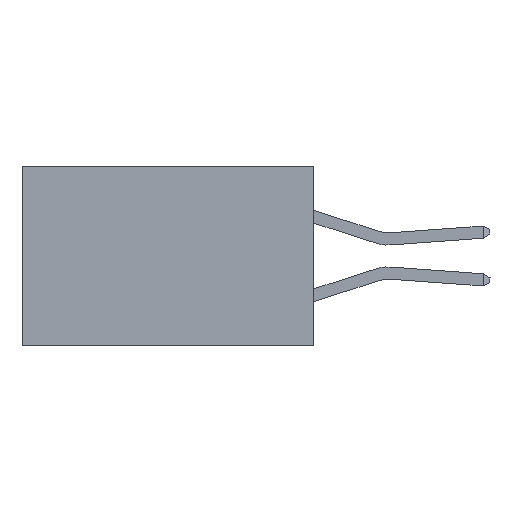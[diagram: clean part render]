
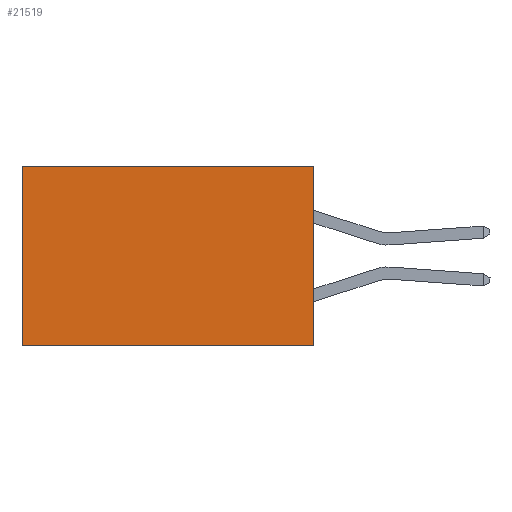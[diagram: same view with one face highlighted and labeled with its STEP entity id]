
A CAD part, left-side view. The second image highlights one B-rep face of the part: STEP entity #21519.
In plain terms, the highlighted planar face has unit normal (-1, 0, 0).
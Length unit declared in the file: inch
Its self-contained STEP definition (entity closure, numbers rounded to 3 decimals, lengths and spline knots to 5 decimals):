
#250 = CARTESIAN_POINT ( 'NONE',  ( 0.2875, 0., -0.37 ) ) ;
#332 = LINE ( 'NONE', #6446, #4777 ) ;
#1845 = VECTOR ( 'NONE', #9595, 39.37008 ) ;
#2243 = DIRECTION ( 'NONE',  ( 1., 0., 0. ) ) ;
#2344 = VERTEX_POINT ( 'NONE', #5003 ) ;
#2877 = VECTOR ( 'NONE', #15956, 39.37008 ) ;
#3766 = EDGE_CURVE ( 'NONE', #2344, #19092, #8052, .T. ) ;
#4233 = DIRECTION ( 'NONE',  ( 0., 0., -1. ) ) ;
#4777 = VECTOR ( 'NONE', #4233, 39.37008 ) ;
#5003 = CARTESIAN_POINT ( 'NONE',  ( 0.2875, 0., 0. ) ) ;
#5112 = ORIENTED_EDGE ( 'NONE', *, *, #9417, .F. ) ;
#6273 = VERTEX_POINT ( 'NONE', #17790 ) ;
#6446 = CARTESIAN_POINT ( 'NONE',  ( 0.2875, 0.6, 0. ) ) ;
#7665 = LINE ( 'NONE', #18468, #1845 ) ;
#8052 = LINE ( 'NONE', #24992, #2877 ) ;
#8468 = EDGE_LOOP ( 'NONE', ( #24601, #5112, #22940, #11428 ) ) ;
#9417 = EDGE_CURVE ( 'NONE', #19092, #25358, #7665, .T. ) ;
#9595 = DIRECTION ( 'NONE',  ( 0., 1., 0. ) ) ;
#11010 = CARTESIAN_POINT ( 'NONE',  ( 0.2875, 0., 0. ) ) ;
#11428 = ORIENTED_EDGE ( 'NONE', *, *, #20713, .T. ) ;
#12634 = DIRECTION ( 'NONE',  ( 0., 1., 0. ) ) ;
#13071 = FACE_OUTER_BOUND ( 'NONE', #8468, .T. ) ;
#13274 = PLANE ( 'NONE',  #24896 ) ;
#15956 = DIRECTION ( 'NONE',  ( 0., 0., -1. ) ) ;
#17151 = CARTESIAN_POINT ( 'NONE',  ( 0.2875, 0., 0. ) ) ;
#17777 = DIRECTION ( 'NONE',  ( 0., 0., -1. ) ) ;
#17790 = CARTESIAN_POINT ( 'NONE',  ( 0.2875, 0.6, 0. ) ) ;
#18468 = CARTESIAN_POINT ( 'NONE',  ( 0.2875, 0., -0.37 ) ) ;
#19092 = VERTEX_POINT ( 'NONE', #250 ) ;
#19624 = EDGE_CURVE ( 'NONE', #6273, #25358, #332, .T. ) ;
#20713 = EDGE_CURVE ( 'NONE', #2344, #6273, #27683, .T. ) ;
#21519 = ADVANCED_FACE ( 'NONE', ( #13071 ), #13274, .F. ) ;
#22940 = ORIENTED_EDGE ( 'NONE', *, *, #3766, .F. ) ;
#24601 = ORIENTED_EDGE ( 'NONE', *, *, #19624, .T. ) ;
#24896 = AXIS2_PLACEMENT_3D ( 'NONE', #11010, #2243, #17777 ) ;
#24992 = CARTESIAN_POINT ( 'NONE',  ( 0.2875, 0., 0. ) ) ;
#25358 = VERTEX_POINT ( 'NONE', #28158 ) ;
#27575 = VECTOR ( 'NONE', #12634, 39.37008 ) ;
#27683 = LINE ( 'NONE', #17151, #27575 ) ;
#28158 = CARTESIAN_POINT ( 'NONE',  ( 0.2875, 0.6, -0.37 ) ) ;
